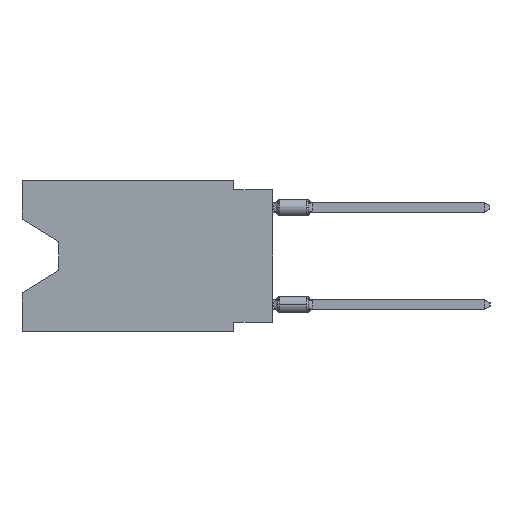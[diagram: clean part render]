
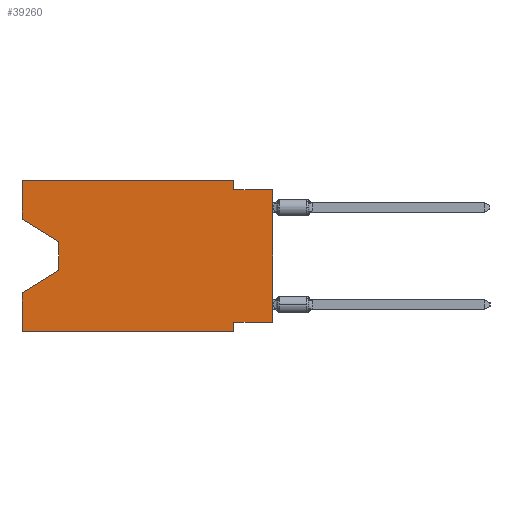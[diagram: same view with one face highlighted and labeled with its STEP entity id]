
A CAD part, left-side view. The second image highlights one B-rep face of the part: STEP entity #39260.
In plain terms, the highlighted planar face has unit normal (-1, 0, 0).
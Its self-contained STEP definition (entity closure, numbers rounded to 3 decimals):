
#512 = VERTEX_POINT ( 'NONE', #12870 ) ;
#1149 = LINE ( 'NONE', #41185, #37866 ) ;
#1556 = VECTOR ( 'NONE', #36859, 1000. ) ;
#1561 = CARTESIAN_POINT ( 'NONE',  ( 0., 0., -0.635 ) ) ;
#3233 = VERTEX_POINT ( 'NONE', #57092 ) ;
#3696 = VECTOR ( 'NONE', #15969, 1000. ) ;
#3745 = AXIS2_PLACEMENT_3D ( 'NONE', #56508, #11587, #31587 ) ;
#4011 = EDGE_CURVE ( 'NONE', #53418, #38337, #1149, .T. ) ;
#5531 = CARTESIAN_POINT ( 'NONE',  ( 0., 0., -9.271 ) ) ;
#6983 = ORIENTED_EDGE ( 'NONE', *, *, #38893, .T. ) ;
#7060 = LINE ( 'NONE', #38249, #47306 ) ;
#8162 = DIRECTION ( 'NONE',  ( 0., 0., 1. ) ) ;
#8618 = ORIENTED_EDGE ( 'NONE', *, *, #46302, .F. ) ;
#9440 = DIRECTION ( 'NONE',  ( 0., -1., 0. ) ) ;
#9822 = LINE ( 'NONE', #55697, #38853 ) ;
#10438 = LINE ( 'NONE', #56718, #55752 ) ;
#11587 = DIRECTION ( 'NONE',  ( 1., 0., 0. ) ) ;
#12150 = EDGE_CURVE ( 'NONE', #3233, #19281, #10438, .T. ) ;
#12870 = CARTESIAN_POINT ( 'NONE',  ( 0., 16.383, 0. ) ) ;
#13096 = CARTESIAN_POINT ( 'NONE',  ( 0., 16.383, 0. ) ) ;
#13153 = EDGE_LOOP ( 'NONE', ( #22694, #18631, #51430, #35751, #6983, #8618, #30783, #42188, #26213, #17969, #57749, #38108 ) ) ;
#14292 = CARTESIAN_POINT ( 'NONE',  ( 0., 2.54, -9.271 ) ) ;
#15077 = LINE ( 'NONE', #34745, #60820 ) ;
#15535 = LINE ( 'NONE', #25702, #50930 ) ;
#15969 = DIRECTION ( 'NONE',  ( 0., -1., 0. ) ) ;
#16022 = LINE ( 'NONE', #1561, #20918 ) ;
#16453 = EDGE_CURVE ( 'NONE', #22412, #17197, #15535, .T. ) ;
#16505 = FACE_OUTER_BOUND ( 'NONE', #13153, .T. ) ;
#17197 = VERTEX_POINT ( 'NONE', #29733 ) ;
#17969 = ORIENTED_EDGE ( 'NONE', *, *, #12150, .F. ) ;
#18631 = ORIENTED_EDGE ( 'NONE', *, *, #26838, .T. ) ;
#19281 = VERTEX_POINT ( 'NONE', #49072 ) ;
#20874 = LINE ( 'NONE', #21860, #3696 ) ;
#20918 = VECTOR ( 'NONE', #25537, 1000. ) ;
#21083 = DIRECTION ( 'NONE',  ( 0., 0.855, -0.519 ) ) ;
#21781 = CARTESIAN_POINT ( 'NONE',  ( 0., 0., -0.635 ) ) ;
#21860 = CARTESIAN_POINT ( 'NONE',  ( 0., 16.383, -9.906 ) ) ;
#22412 = VERTEX_POINT ( 'NONE', #47709 ) ;
#22694 = ORIENTED_EDGE ( 'NONE', *, *, #4011, .T. ) ;
#25494 = LINE ( 'NONE', #49782, #53127 ) ;
#25537 = DIRECTION ( 'NONE',  ( 0., -1., 0. ) ) ;
#25702 = CARTESIAN_POINT ( 'NONE',  ( 0., 13.97, -5.893 ) ) ;
#26213 = ORIENTED_EDGE ( 'NONE', *, *, #44586, .F. ) ;
#26822 = EDGE_CURVE ( 'NONE', #28682, #17197, #15077, .T. ) ;
#26838 = EDGE_CURVE ( 'NONE', #38337, #22412, #9822, .T. ) ;
#28228 = CARTESIAN_POINT ( 'NONE',  ( 0., 16.383, -9.906 ) ) ;
#28682 = VERTEX_POINT ( 'NONE', #28228 ) ;
#29733 = CARTESIAN_POINT ( 'NONE',  ( 0., 16.383, -7.36 ) ) ;
#29821 = DIRECTION ( 'NONE',  ( 0., 0., -1. ) ) ;
#30459 = LINE ( 'NONE', #5531, #52994 ) ;
#30783 = ORIENTED_EDGE ( 'NONE', *, *, #31789, .F. ) ;
#31587 = DIRECTION ( 'NONE',  ( 0., 0., -1. ) ) ;
#31789 = EDGE_CURVE ( 'NONE', #63223, #40654, #30459, .T. ) ;
#32769 = EDGE_CURVE ( 'NONE', #63223, #40885, #46361, .T. ) ;
#33307 = DIRECTION ( 'NONE',  ( 0., 0., -1. ) ) ;
#33565 = CARTESIAN_POINT ( 'NONE',  ( 0., 13.97, -4.013 ) ) ;
#34745 = CARTESIAN_POINT ( 'NONE',  ( 0., 16.383, 0. ) ) ;
#35087 = EDGE_CURVE ( 'NONE', #512, #3233, #25494, .T. ) ;
#35751 = ORIENTED_EDGE ( 'NONE', *, *, #26822, .F. ) ;
#36522 = PLANE ( 'NONE',  #3745 ) ;
#36859 = DIRECTION ( 'NONE',  ( 0., 0., 1. ) ) ;
#37866 = VECTOR ( 'NONE', #61188, 1000. ) ;
#38108 = ORIENTED_EDGE ( 'NONE', *, *, #41685, .F. ) ;
#38249 = CARTESIAN_POINT ( 'NONE',  ( 0., 2.54, -9.906 ) ) ;
#38337 = VERTEX_POINT ( 'NONE', #33565 ) ;
#38346 = LINE ( 'NONE', #13096, #61665 ) ;
#38853 = VECTOR ( 'NONE', #29821, 1000. ) ;
#38893 = EDGE_CURVE ( 'NONE', #28682, #41393, #20874, .T. ) ;
#39260 = ADVANCED_FACE ( 'NONE', ( #16505 ), #36522, .F. ) ;
#40654 = VERTEX_POINT ( 'NONE', #14292 ) ;
#40885 = VERTEX_POINT ( 'NONE', #21781 ) ;
#40992 = CARTESIAN_POINT ( 'NONE',  ( 0., 0., -9.271 ) ) ;
#41185 = CARTESIAN_POINT ( 'NONE',  ( 0., 16.383, -2.546 ) ) ;
#41257 = DIRECTION ( 'NONE',  ( 0., 0., -1. ) ) ;
#41393 = VERTEX_POINT ( 'NONE', #43351 ) ;
#41685 = EDGE_CURVE ( 'NONE', #53418, #512, #38346, .T. ) ;
#41771 = CARTESIAN_POINT ( 'NONE',  ( 0., 0., 0. ) ) ;
#42188 = ORIENTED_EDGE ( 'NONE', *, *, #32769, .T. ) ;
#43351 = CARTESIAN_POINT ( 'NONE',  ( 0., 2.54, -9.906 ) ) ;
#44586 = EDGE_CURVE ( 'NONE', #19281, #40885, #16022, .T. ) ;
#46302 = EDGE_CURVE ( 'NONE', #40654, #41393, #7060, .T. ) ;
#46361 = LINE ( 'NONE', #41771, #1556 ) ;
#47306 = VECTOR ( 'NONE', #33307, 1000. ) ;
#47709 = CARTESIAN_POINT ( 'NONE',  ( 0., 13.97, -5.893 ) ) ;
#49072 = CARTESIAN_POINT ( 'NONE',  ( 0., 2.54, -0.635 ) ) ;
#49782 = CARTESIAN_POINT ( 'NONE',  ( 0., 16.383, 0. ) ) ;
#50930 = VECTOR ( 'NONE', #21083, 1000. ) ;
#51425 = DIRECTION ( 'NONE',  ( 0., 1., 0. ) ) ;
#51430 = ORIENTED_EDGE ( 'NONE', *, *, #16453, .T. ) ;
#52994 = VECTOR ( 'NONE', #51425, 1000. ) ;
#53127 = VECTOR ( 'NONE', #9440, 1000. ) ;
#53418 = VERTEX_POINT ( 'NONE', #64691 ) ;
#55697 = CARTESIAN_POINT ( 'NONE',  ( 0., 13.97, -4.013 ) ) ;
#55752 = VECTOR ( 'NONE', #41257, 1000. ) ;
#56508 = CARTESIAN_POINT ( 'NONE',  ( 0., 16.383, 0. ) ) ;
#56718 = CARTESIAN_POINT ( 'NONE',  ( 0., 2.54, 0. ) ) ;
#57092 = CARTESIAN_POINT ( 'NONE',  ( 0., 2.54, 0. ) ) ;
#57749 = ORIENTED_EDGE ( 'NONE', *, *, #35087, .F. ) ;
#59653 = DIRECTION ( 'NONE',  ( 0., 0., 1. ) ) ;
#60820 = VECTOR ( 'NONE', #59653, 1000. ) ;
#61188 = DIRECTION ( 'NONE',  ( 0., -0.855, -0.519 ) ) ;
#61665 = VECTOR ( 'NONE', #8162, 1000. ) ;
#63223 = VERTEX_POINT ( 'NONE', #40992 ) ;
#64691 = CARTESIAN_POINT ( 'NONE',  ( 0., 16.383, -2.546 ) ) ;
